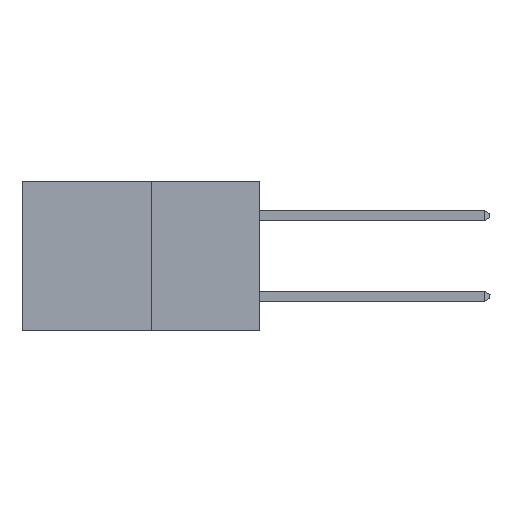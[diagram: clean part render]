
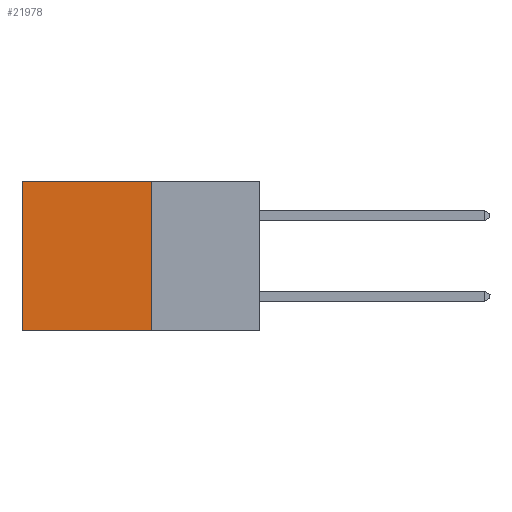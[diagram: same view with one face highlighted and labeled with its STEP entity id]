
A CAD part, left-side view. The second image highlights one B-rep face of the part: STEP entity #21978.
In plain terms, the highlighted planar face has unit normal (-1, 0, 0).
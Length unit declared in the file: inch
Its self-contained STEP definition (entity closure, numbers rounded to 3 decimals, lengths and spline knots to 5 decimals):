
#2 = CARTESIAN_POINT ( 'NONE',  ( 0.277, 0.27, 0. ) ) ;
#53 = CARTESIAN_POINT ( 'NONE',  ( 0.277, 0.59, -0.37 ) ) ;
#404 = EDGE_CURVE ( 'NONE', #5665, #20562, #9447, .T. ) ;
#544 = CARTESIAN_POINT ( 'NONE',  ( 0.277, 0.59, 0. ) ) ;
#1023 = DIRECTION ( 'NONE',  ( 0., 0., -1. ) ) ;
#3302 = LINE ( 'NONE', #18103, #13059 ) ;
#4523 = FACE_OUTER_BOUND ( 'NONE', #19813, .T. ) ;
#4637 = CARTESIAN_POINT ( 'NONE',  ( 0.277, 0.27, 0. ) ) ;
#4830 = VECTOR ( 'NONE', #7623, 39.37008 ) ;
#5660 = VERTEX_POINT ( 'NONE', #53 ) ;
#5665 = VERTEX_POINT ( 'NONE', #2 ) ;
#6060 = DIRECTION ( 'NONE',  ( 0., 0., -1. ) ) ;
#6444 = LINE ( 'NONE', #15225, #13966 ) ;
#6655 = DIRECTION ( 'NONE',  ( 0., 1., 0. ) ) ;
#7082 = EDGE_CURVE ( 'NONE', #20562, #5660, #16298, .T. ) ;
#7623 = DIRECTION ( 'NONE',  ( 0., 1., 0. ) ) ;
#9447 = LINE ( 'NONE', #4637, #4830 ) ;
#9691 = PLANE ( 'NONE',  #16003 ) ;
#10399 = ORIENTED_EDGE ( 'NONE', *, *, #18046, .F. ) ;
#10413 = DIRECTION ( 'NONE',  ( 0., 0., -1. ) ) ;
#11085 = EDGE_CURVE ( 'NONE', #12810, #5660, #6444, .T. ) ;
#11423 = DIRECTION ( 'NONE',  ( 1., 0., 0. ) ) ;
#11569 = ORIENTED_EDGE ( 'NONE', *, *, #11085, .F. ) ;
#12810 = VERTEX_POINT ( 'NONE', #15288 ) ;
#13059 = VECTOR ( 'NONE', #6060, 39.37008 ) ;
#13966 = VECTOR ( 'NONE', #6655, 39.37008 ) ;
#15225 = CARTESIAN_POINT ( 'NONE',  ( 0.277, 0.27, -0.37 ) ) ;
#15239 = ORIENTED_EDGE ( 'NONE', *, *, #7082, .T. ) ;
#15288 = CARTESIAN_POINT ( 'NONE',  ( 0.277, 0.27, -0.37 ) ) ;
#16003 = AXIS2_PLACEMENT_3D ( 'NONE', #20017, #11423, #1023 ) ;
#16298 = LINE ( 'NONE', #18998, #20915 ) ;
#18046 = EDGE_CURVE ( 'NONE', #5665, #12810, #3302, .T. ) ;
#18103 = CARTESIAN_POINT ( 'NONE',  ( 0.277, 0.27, -0.37 ) ) ;
#18998 = CARTESIAN_POINT ( 'NONE',  ( 0.277, 0.59, -0.37 ) ) ;
#19813 = EDGE_LOOP ( 'NONE', ( #15239, #11569, #10399, #20916 ) ) ;
#20017 = CARTESIAN_POINT ( 'NONE',  ( 0.277, 0.27, -0.37 ) ) ;
#20562 = VERTEX_POINT ( 'NONE', #544 ) ;
#20915 = VECTOR ( 'NONE', #10413, 39.37008 ) ;
#20916 = ORIENTED_EDGE ( 'NONE', *, *, #404, .T. ) ;
#21978 = ADVANCED_FACE ( 'NONE', ( #4523 ), #9691, .F. ) ;
